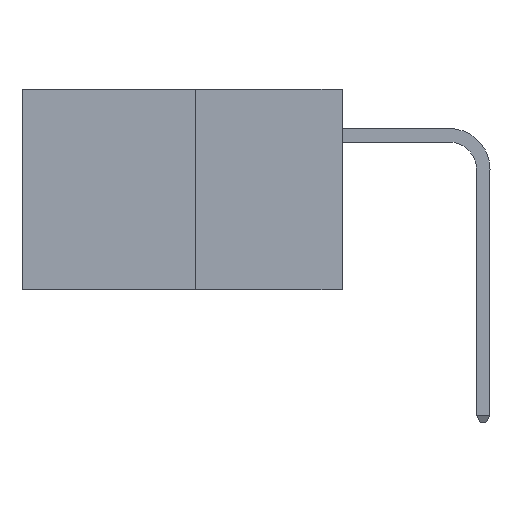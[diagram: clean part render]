
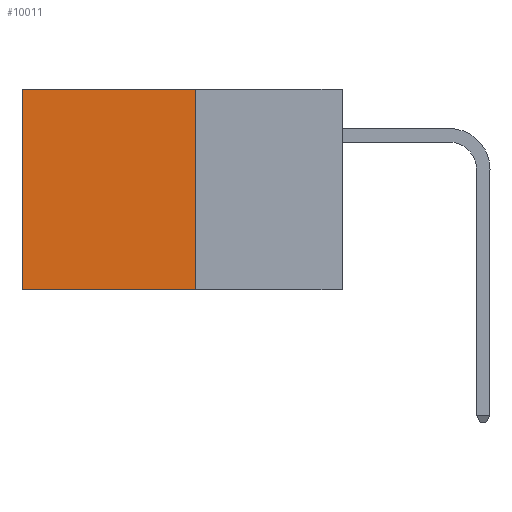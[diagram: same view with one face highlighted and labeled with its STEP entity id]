
A CAD part, left-side view. The second image highlights one B-rep face of the part: STEP entity #10011.
In plain terms, the highlighted planar face has unit normal (-1, 0, 0).
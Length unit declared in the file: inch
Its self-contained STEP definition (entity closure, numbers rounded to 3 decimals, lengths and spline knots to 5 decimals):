
#45 = ORIENTED_EDGE ( 'NONE', *, *, #12751, .T. ) ;
#370 = LINE ( 'NONE', #14947, #12618 ) ;
#397 = LINE ( 'NONE', #10891, #8911 ) ;
#1573 = DIRECTION ( 'NONE',  ( 0., 0., -1. ) ) ;
#1631 = VECTOR ( 'NONE', #2936, 39.37008 ) ;
#1734 = VERTEX_POINT ( 'NONE', #14460 ) ;
#2501 = ORIENTED_EDGE ( 'NONE', *, *, #15218, .T. ) ;
#2936 = DIRECTION ( 'NONE',  ( 0., 1., 0. ) ) ;
#3153 = ORIENTED_EDGE ( 'NONE', *, *, #8595, .F. ) ;
#3563 = CARTESIAN_POINT ( 'NONE',  ( 0.277, 0.27, 0. ) ) ;
#4104 = EDGE_LOOP ( 'NONE', ( #2501, #6923, #3153, #45 ) ) ;
#4223 = EDGE_CURVE ( 'NONE', #13018, #14291, #397, .T. ) ;
#6923 = ORIENTED_EDGE ( 'NONE', *, *, #4223, .F. ) ;
#7144 = VERTEX_POINT ( 'NONE', #3563 ) ;
#7549 = LINE ( 'NONE', #10256, #11811 ) ;
#8595 = EDGE_CURVE ( 'NONE', #7144, #13018, #7549, .T. ) ;
#8613 = DIRECTION ( 'NONE',  ( 0., 0., -1. ) ) ;
#8911 = VECTOR ( 'NONE', #10938, 39.37008 ) ;
#9905 = DIRECTION ( 'NONE',  ( 0., 0., -1. ) ) ;
#10011 = ADVANCED_FACE ( 'NONE', ( #12988 ), #15854, .F. ) ;
#10256 = CARTESIAN_POINT ( 'NONE',  ( 0.277, 0.27, -0.37 ) ) ;
#10891 = CARTESIAN_POINT ( 'NONE',  ( 0.277, 0.27, -0.37 ) ) ;
#10938 = DIRECTION ( 'NONE',  ( 0., 1., 0. ) ) ;
#11165 = DIRECTION ( 'NONE',  ( 1., 0., 0. ) ) ;
#11437 = CARTESIAN_POINT ( 'NONE',  ( 0.277, 0.27, -0.37 ) ) ;
#11811 = VECTOR ( 'NONE', #9905, 39.37008 ) ;
#12618 = VECTOR ( 'NONE', #8613, 39.37008 ) ;
#12751 = EDGE_CURVE ( 'NONE', #7144, #1734, #14888, .T. ) ;
#12988 = FACE_OUTER_BOUND ( 'NONE', #4104, .T. ) ;
#13018 = VERTEX_POINT ( 'NONE', #11437 ) ;
#14291 = VERTEX_POINT ( 'NONE', #19481 ) ;
#14460 = CARTESIAN_POINT ( 'NONE',  ( 0.277, 0.59, 0. ) ) ;
#14888 = LINE ( 'NONE', #17212, #1631 ) ;
#14947 = CARTESIAN_POINT ( 'NONE',  ( 0.277, 0.59, -0.37 ) ) ;
#15218 = EDGE_CURVE ( 'NONE', #1734, #14291, #370, .T. ) ;
#15854 = PLANE ( 'NONE',  #16701 ) ;
#16701 = AXIS2_PLACEMENT_3D ( 'NONE', #18966, #11165, #1573 ) ;
#17212 = CARTESIAN_POINT ( 'NONE',  ( 0.277, 0.27, 0. ) ) ;
#18966 = CARTESIAN_POINT ( 'NONE',  ( 0.277, 0.27, -0.37 ) ) ;
#19481 = CARTESIAN_POINT ( 'NONE',  ( 0.277, 0.59, -0.37 ) ) ;
